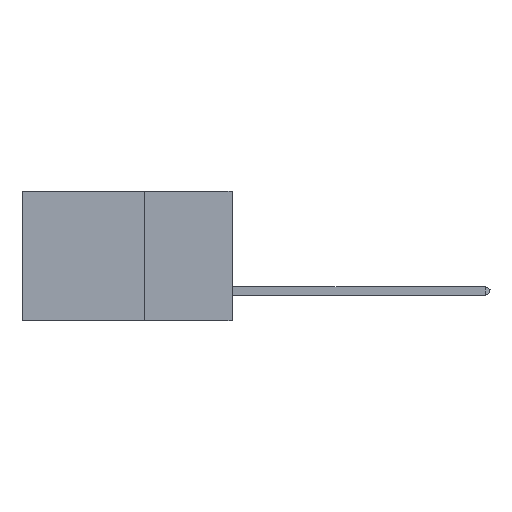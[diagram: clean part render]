
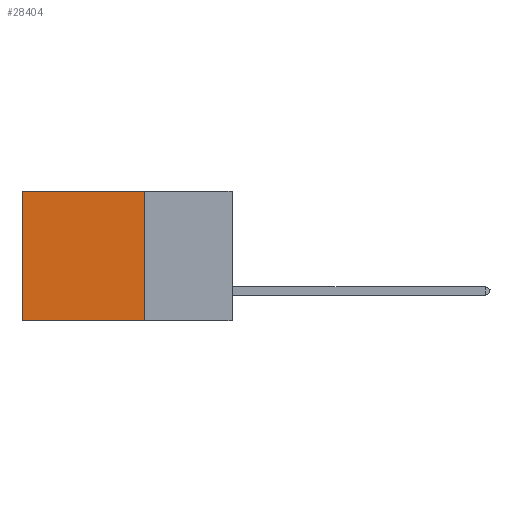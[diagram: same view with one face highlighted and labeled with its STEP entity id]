
A CAD part, left-side view. The second image highlights one B-rep face of the part: STEP entity #28404.
In plain terms, the highlighted planar face has unit normal (-1, 0, 0).
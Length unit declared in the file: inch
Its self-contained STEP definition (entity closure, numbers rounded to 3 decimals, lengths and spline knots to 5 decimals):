
#1787 = VECTOR ( 'NONE', #39293, 39.37008 ) ;
#2095 = CARTESIAN_POINT ( 'NONE',  ( 0.2875, 0.25, 0. ) ) ;
#3734 = CARTESIAN_POINT ( 'NONE',  ( 0.2875, 0.6, 0. ) ) ;
#4879 = CARTESIAN_POINT ( 'NONE',  ( 0.2875, 0.25, -0.37 ) ) ;
#5540 = FACE_OUTER_BOUND ( 'NONE', #7022, .T. ) ;
#5788 = LINE ( 'NONE', #2095, #36058 ) ;
#7022 = EDGE_LOOP ( 'NONE', ( #31509, #10769, #26526, #35414 ) ) ;
#7122 = CARTESIAN_POINT ( 'NONE',  ( 0.2875, 0.6, -0.37 ) ) ;
#7362 = AXIS2_PLACEMENT_3D ( 'NONE', #39723, #30152, #10462 ) ;
#8103 = EDGE_CURVE ( 'NONE', #16832, #30918, #14611, .T. ) ;
#9118 = DIRECTION ( 'NONE',  ( 0., 0., -1. ) ) ;
#10462 = DIRECTION ( 'NONE',  ( 0., 0., -1. ) ) ;
#10588 = PLANE ( 'NONE',  #7362 ) ;
#10769 = ORIENTED_EDGE ( 'NONE', *, *, #8103, .F. ) ;
#12720 = EDGE_CURVE ( 'NONE', #21706, #30918, #16753, .T. ) ;
#13044 = CARTESIAN_POINT ( 'NONE',  ( 0.2875, 0.25, -0.37 ) ) ;
#14611 = LINE ( 'NONE', #13044, #1787 ) ;
#16753 = LINE ( 'NONE', #17083, #24478 ) ;
#16832 = VERTEX_POINT ( 'NONE', #4879 ) ;
#17083 = CARTESIAN_POINT ( 'NONE',  ( 0.2875, 0.6, 0. ) ) ;
#21706 = VERTEX_POINT ( 'NONE', #3734 ) ;
#23152 = LINE ( 'NONE', #34370, #32414 ) ;
#24478 = VECTOR ( 'NONE', #28031, 39.37008 ) ;
#26526 = ORIENTED_EDGE ( 'NONE', *, *, #39247, .F. ) ;
#27645 = DIRECTION ( 'NONE',  ( 0., 1., 0. ) ) ;
#27674 = VERTEX_POINT ( 'NONE', #42351 ) ;
#28031 = DIRECTION ( 'NONE',  ( 0., 0., -1. ) ) ;
#28404 = ADVANCED_FACE ( 'NONE', ( #5540 ), #10588, .F. ) ;
#30152 = DIRECTION ( 'NONE',  ( 1., 0., 0. ) ) ;
#30918 = VERTEX_POINT ( 'NONE', #7122 ) ;
#31509 = ORIENTED_EDGE ( 'NONE', *, *, #12720, .T. ) ;
#32317 = EDGE_CURVE ( 'NONE', #27674, #21706, #23152, .T. ) ;
#32414 = VECTOR ( 'NONE', #27645, 39.37008 ) ;
#34370 = CARTESIAN_POINT ( 'NONE',  ( 0.2875, 0.25, 0. ) ) ;
#35414 = ORIENTED_EDGE ( 'NONE', *, *, #32317, .T. ) ;
#36058 = VECTOR ( 'NONE', #9118, 39.37008 ) ;
#39247 = EDGE_CURVE ( 'NONE', #27674, #16832, #5788, .T. ) ;
#39293 = DIRECTION ( 'NONE',  ( 0., 1., 0. ) ) ;
#39723 = CARTESIAN_POINT ( 'NONE',  ( 0.2875, 0.25, 0. ) ) ;
#42351 = CARTESIAN_POINT ( 'NONE',  ( 0.2875, 0.25, 0. ) ) ;
